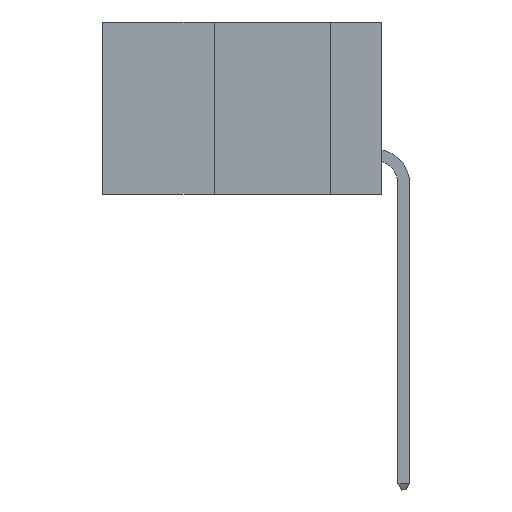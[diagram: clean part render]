
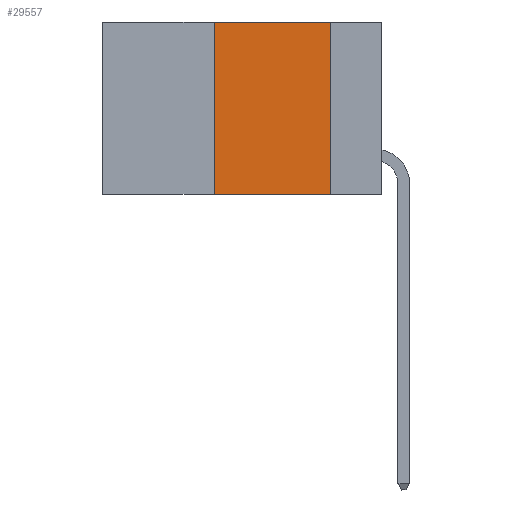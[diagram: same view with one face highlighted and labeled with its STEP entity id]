
A CAD part, left-side view. The second image highlights one B-rep face of the part: STEP entity #29557.
In plain terms, the highlighted planar face has unit normal (-1, 0, 0).
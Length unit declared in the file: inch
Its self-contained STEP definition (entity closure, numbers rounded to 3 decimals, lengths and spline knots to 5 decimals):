
#217 = VERTEX_POINT ( 'NONE', #26895 ) ;
#2460 = LINE ( 'NONE', #16883, #11522 ) ;
#2719 = ORIENTED_EDGE ( 'NONE', *, *, #31088, .T. ) ;
#7075 = CARTESIAN_POINT ( 'NONE',  ( 0., 0.6, -0.37 ) ) ;
#7260 = CARTESIAN_POINT ( 'NONE',  ( 0., 0.11, -0.37 ) ) ;
#7275 = EDGE_CURVE ( 'NONE', #20449, #28803, #8445, .T. ) ;
#7866 = CARTESIAN_POINT ( 'NONE',  ( 0., 0.11, 0. ) ) ;
#8445 = LINE ( 'NONE', #7866, #28824 ) ;
#9792 = DIRECTION ( 'NONE',  ( 0., 0., -1. ) ) ;
#11522 = VECTOR ( 'NONE', #21563, 39.37008 ) ;
#12314 = PLANE ( 'NONE',  #23087 ) ;
#12700 = VECTOR ( 'NONE', #29419, 39.37008 ) ;
#15463 = VECTOR ( 'NONE', #27401, 39.37008 ) ;
#16678 = ORIENTED_EDGE ( 'NONE', *, *, #17829, .F. ) ;
#16883 = CARTESIAN_POINT ( 'NONE',  ( 0., 0.36, 0. ) ) ;
#17035 = CARTESIAN_POINT ( 'NONE',  ( 0., 0.6, 0. ) ) ;
#17829 = EDGE_CURVE ( 'NONE', #217, #20449, #18225, .T. ) ;
#18225 = LINE ( 'NONE', #17035, #15463 ) ;
#18317 = DIRECTION ( 'NONE',  ( 0., 0., -1. ) ) ;
#18565 = LINE ( 'NONE', #7075, #12700 ) ;
#18794 = ORIENTED_EDGE ( 'NONE', *, *, #22165, .F. ) ;
#20170 = CARTESIAN_POINT ( 'NONE',  ( 0., 0.11, 0. ) ) ;
#20254 = FACE_OUTER_BOUND ( 'NONE', #28548, .T. ) ;
#20449 = VERTEX_POINT ( 'NONE', #20170 ) ;
#21563 = DIRECTION ( 'NONE',  ( 0., 0., 1. ) ) ;
#22157 = DIRECTION ( 'NONE',  ( 1., 0., 0. ) ) ;
#22165 = EDGE_CURVE ( 'NONE', #25218, #217, #2460, .T. ) ;
#23087 = AXIS2_PLACEMENT_3D ( 'NONE', #32378, #22157, #9792 ) ;
#23951 = CARTESIAN_POINT ( 'NONE',  ( 0., 0.36, -0.37 ) ) ;
#25218 = VERTEX_POINT ( 'NONE', #23951 ) ;
#26153 = ORIENTED_EDGE ( 'NONE', *, *, #7275, .F. ) ;
#26895 = CARTESIAN_POINT ( 'NONE',  ( 0., 0.36, 0. ) ) ;
#27401 = DIRECTION ( 'NONE',  ( 0., -1., 0. ) ) ;
#28548 = EDGE_LOOP ( 'NONE', ( #26153, #16678, #18794, #2719 ) ) ;
#28803 = VERTEX_POINT ( 'NONE', #7260 ) ;
#28824 = VECTOR ( 'NONE', #18317, 39.37008 ) ;
#29419 = DIRECTION ( 'NONE',  ( 0., -1., 0. ) ) ;
#29557 = ADVANCED_FACE ( 'NONE', ( #20254 ), #12314, .F. ) ;
#31088 = EDGE_CURVE ( 'NONE', #25218, #28803, #18565, .T. ) ;
#32378 = CARTESIAN_POINT ( 'NONE',  ( 0., 0.6, 0. ) ) ;
